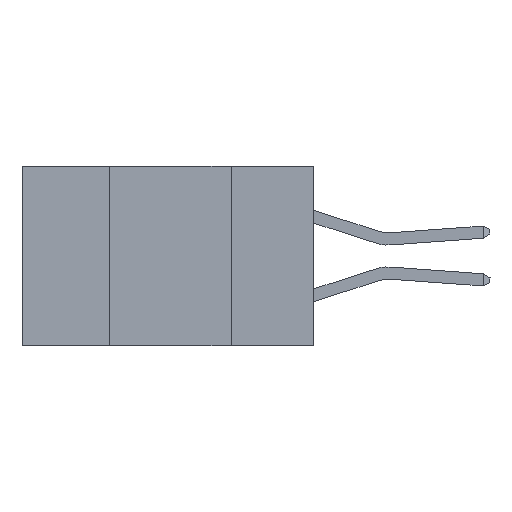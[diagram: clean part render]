
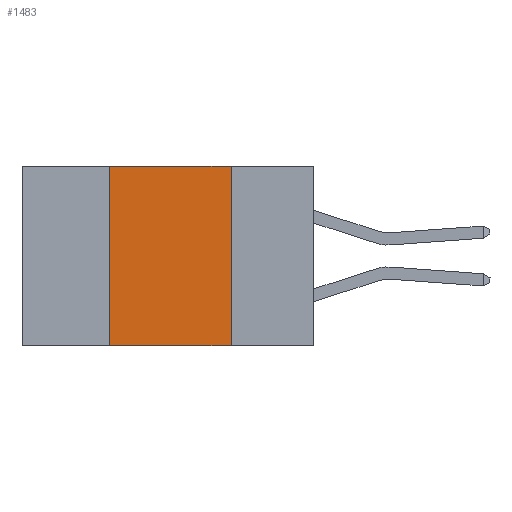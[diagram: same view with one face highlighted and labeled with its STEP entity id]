
A CAD part, left-side view. The second image highlights one B-rep face of the part: STEP entity #1483.
In plain terms, the highlighted planar face has unit normal (-1, 0, 0).
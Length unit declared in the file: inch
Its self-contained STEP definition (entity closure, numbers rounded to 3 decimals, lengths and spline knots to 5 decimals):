
#355 = LINE ( 'NONE', #12708, #21028 ) ;
#430 = CARTESIAN_POINT ( 'NONE',  ( 0., 0.17, 0. ) ) ;
#590 = LINE ( 'NONE', #430, #2991 ) ;
#751 = DIRECTION ( 'NONE',  ( 0., 0., 1. ) ) ;
#1483 = ADVANCED_FACE ( 'NONE', ( #6797 ), #14653, .F. ) ;
#1648 = DIRECTION ( 'NONE',  ( 0., -1., 0. ) ) ;
#2432 = VERTEX_POINT ( 'NONE', #19797 ) ;
#2597 = EDGE_CURVE ( 'NONE', #22815, #9688, #18510, .T. ) ;
#2915 = EDGE_CURVE ( 'NONE', #17447, #2432, #355, .T. ) ;
#2991 = VECTOR ( 'NONE', #15369, 39.37008 ) ;
#6797 = FACE_OUTER_BOUND ( 'NONE', #14870, .T. ) ;
#9688 = VERTEX_POINT ( 'NONE', #18298 ) ;
#10365 = CARTESIAN_POINT ( 'NONE',  ( 0., 0.42, 0. ) ) ;
#11940 = EDGE_CURVE ( 'NONE', #22815, #17447, #27366, .T. ) ;
#12078 = ORIENTED_EDGE ( 'NONE', *, *, #11940, .F. ) ;
#12708 = CARTESIAN_POINT ( 'NONE',  ( 0., 0.6, 0. ) ) ;
#14653 = PLANE ( 'NONE',  #18816 ) ;
#14870 = EDGE_LOOP ( 'NONE', ( #26488, #20134, #12078, #26262 ) ) ;
#15369 = DIRECTION ( 'NONE',  ( 0., 0., -1. ) ) ;
#15837 = VECTOR ( 'NONE', #751, 39.37008 ) ;
#15909 = VECTOR ( 'NONE', #1648, 39.37008 ) ;
#16121 = CARTESIAN_POINT ( 'NONE',  ( 0., 0.42, 0. ) ) ;
#17447 = VERTEX_POINT ( 'NONE', #16121 ) ;
#17512 = DIRECTION ( 'NONE',  ( 0., -1., 0. ) ) ;
#18298 = CARTESIAN_POINT ( 'NONE',  ( 0., 0.17, -0.37 ) ) ;
#18510 = LINE ( 'NONE', #23471, #15909 ) ;
#18816 = AXIS2_PLACEMENT_3D ( 'NONE', #31322, #24416, #29221 ) ;
#19797 = CARTESIAN_POINT ( 'NONE',  ( 0., 0.17, 0. ) ) ;
#20134 = ORIENTED_EDGE ( 'NONE', *, *, #2915, .F. ) ;
#21028 = VECTOR ( 'NONE', #17512, 39.37008 ) ;
#21165 = CARTESIAN_POINT ( 'NONE',  ( 0., 0.42, -0.37 ) ) ;
#22815 = VERTEX_POINT ( 'NONE', #21165 ) ;
#23471 = CARTESIAN_POINT ( 'NONE',  ( 0., 0.6, -0.37 ) ) ;
#24416 = DIRECTION ( 'NONE',  ( 1., 0., 0. ) ) ;
#26262 = ORIENTED_EDGE ( 'NONE', *, *, #2597, .T. ) ;
#26488 = ORIENTED_EDGE ( 'NONE', *, *, #28041, .F. ) ;
#27366 = LINE ( 'NONE', #10365, #15837 ) ;
#28041 = EDGE_CURVE ( 'NONE', #2432, #9688, #590, .T. ) ;
#29221 = DIRECTION ( 'NONE',  ( 0., 0., -1. ) ) ;
#31322 = CARTESIAN_POINT ( 'NONE',  ( 0., 0.6, 0. ) ) ;
